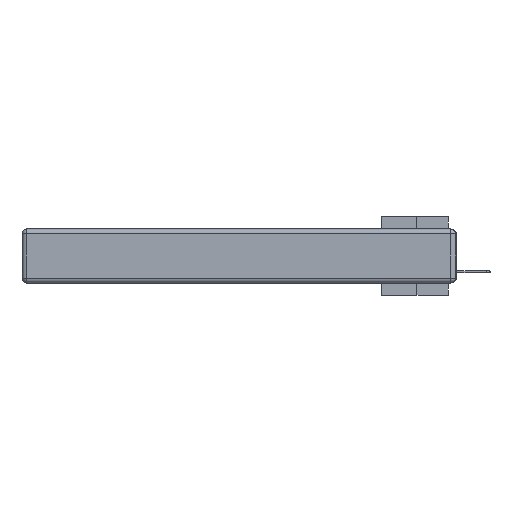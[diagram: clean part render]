
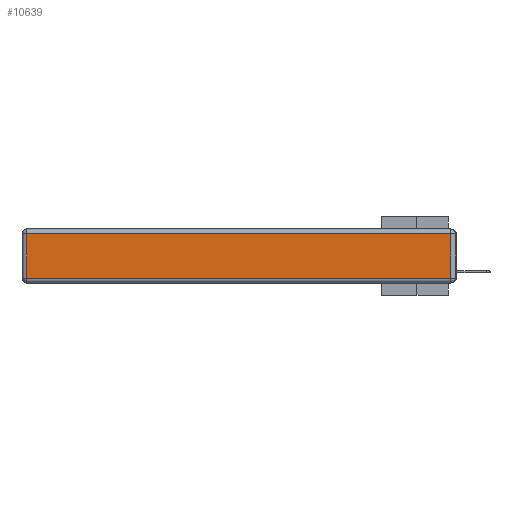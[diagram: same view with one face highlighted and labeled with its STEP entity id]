
A CAD part, left-side view. The second image highlights one B-rep face of the part: STEP entity #10639.
In plain terms, the highlighted planar face has unit normal (-1, 0, 0).
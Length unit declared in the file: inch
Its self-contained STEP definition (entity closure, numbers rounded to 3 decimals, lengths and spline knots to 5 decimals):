
#1620 = DIRECTION ( 'NONE',  ( 0., 0., 1. ) ) ;
#2051 = LINE ( 'NONE', #24110, #11468 ) ;
#2423 = ORIENTED_EDGE ( 'NONE', *, *, #2503, .T. ) ;
#2503 = EDGE_CURVE ( 'NONE', #10658, #8628, #2051, .T. ) ;
#2875 = VECTOR ( 'NONE', #13572, 39.37008 ) ;
#3022 = VECTOR ( 'NONE', #21146, 39.37008 ) ;
#3268 = VERTEX_POINT ( 'NONE', #31390 ) ;
#6409 = FACE_OUTER_BOUND ( 'NONE', #12325, .T. ) ;
#6668 = ORIENTED_EDGE ( 'NONE', *, *, #27236, .T. ) ;
#8388 = EDGE_CURVE ( 'NONE', #3268, #10754, #33063, .T. ) ;
#8628 = VERTEX_POINT ( 'NONE', #32686 ) ;
#9000 = EDGE_CURVE ( 'NONE', #8628, #3268, #24530, .T. ) ;
#9921 = AXIS2_PLACEMENT_3D ( 'NONE', #33547, #17788, #1620 ) ;
#10639 = ADVANCED_FACE ( 'NONE', ( #6409 ), #28078, .T. ) ;
#10658 = VERTEX_POINT ( 'NONE', #28424 ) ;
#10754 = VERTEX_POINT ( 'NONE', #20816 ) ;
#11468 = VECTOR ( 'NONE', #13060, 39.37008 ) ;
#12325 = EDGE_LOOP ( 'NONE', ( #16190, #18762, #6668, #2423 ) ) ;
#13060 = DIRECTION ( 'NONE',  ( 0., 0., -1. ) ) ;
#13572 = DIRECTION ( 'NONE',  ( 0., 1., 0. ) ) ;
#14778 = CARTESIAN_POINT ( 'NONE',  ( 0., 0.03, -0.343 ) ) ;
#16190 = ORIENTED_EDGE ( 'NONE', *, *, #9000, .T. ) ;
#16589 = LINE ( 'NONE', #33055, #2875 ) ;
#16764 = DIRECTION ( 'NONE',  ( 0., 0., 1. ) ) ;
#17788 = DIRECTION ( 'NONE',  ( -1., 0., 0. ) ) ;
#18762 = ORIENTED_EDGE ( 'NONE', *, *, #8388, .T. ) ;
#20816 = CARTESIAN_POINT ( 'NONE',  ( 0., 0.03, -0.03 ) ) ;
#21146 = DIRECTION ( 'NONE',  ( 0., -1., 0. ) ) ;
#24110 = CARTESIAN_POINT ( 'NONE',  ( 0., 2.72, -0.343 ) ) ;
#24530 = LINE ( 'NONE', #26650, #3022 ) ;
#26650 = CARTESIAN_POINT ( 'NONE',  ( 0., 0., -0.313 ) ) ;
#27236 = EDGE_CURVE ( 'NONE', #10754, #10658, #16589, .T. ) ;
#28004 = VECTOR ( 'NONE', #16764, 39.37008 ) ;
#28078 = PLANE ( 'NONE',  #9921 ) ;
#28424 = CARTESIAN_POINT ( 'NONE',  ( 0., 2.72, -0.03 ) ) ;
#31390 = CARTESIAN_POINT ( 'NONE',  ( 0., 0.03, -0.313 ) ) ;
#32686 = CARTESIAN_POINT ( 'NONE',  ( 0., 2.72, -0.313 ) ) ;
#33055 = CARTESIAN_POINT ( 'NONE',  ( 0., 2.75, -0.03 ) ) ;
#33063 = LINE ( 'NONE', #14778, #28004 ) ;
#33547 = CARTESIAN_POINT ( 'NONE',  ( 0., 0., -0.343 ) ) ;
